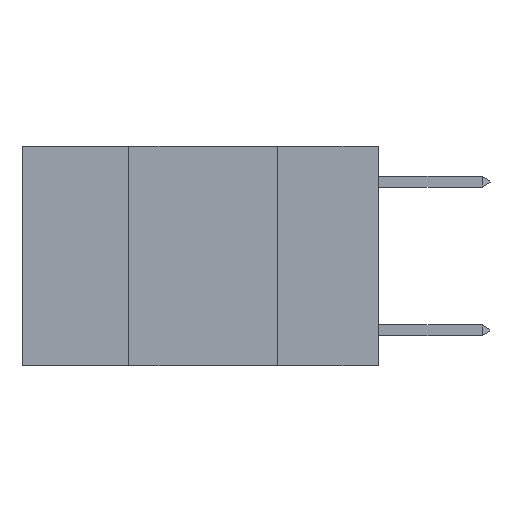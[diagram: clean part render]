
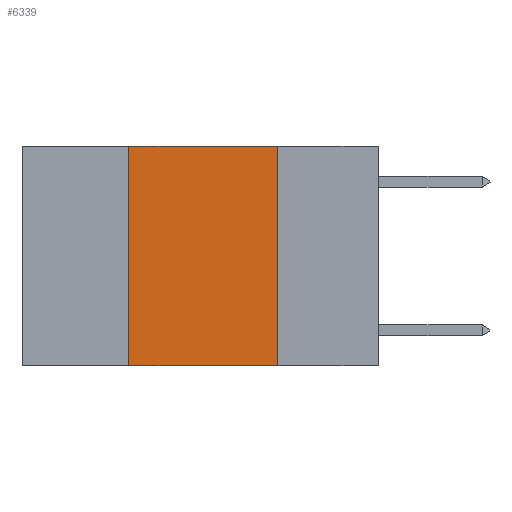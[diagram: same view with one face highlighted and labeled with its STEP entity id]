
A CAD part, left-side view. The second image highlights one B-rep face of the part: STEP entity #6339.
In plain terms, the highlighted planar face has unit normal (-1, 0, 0).
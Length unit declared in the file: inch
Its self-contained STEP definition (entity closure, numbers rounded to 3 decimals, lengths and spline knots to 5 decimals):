
#99 = CARTESIAN_POINT ( 'NONE',  ( 0., 0.6, -0.37 ) ) ;
#172 = EDGE_CURVE ( 'NONE', #1298, #14759, #4029, .T. ) ;
#753 = CARTESIAN_POINT ( 'NONE',  ( 0., 0.42, 0. ) ) ;
#875 = VECTOR ( 'NONE', #6077, 39.37008 ) ;
#1265 = ORIENTED_EDGE ( 'NONE', *, *, #14210, .F. ) ;
#1298 = VERTEX_POINT ( 'NONE', #15104 ) ;
#1406 = CARTESIAN_POINT ( 'NONE',  ( 0., 0.17, 0. ) ) ;
#1576 = VERTEX_POINT ( 'NONE', #1579 ) ;
#1579 = CARTESIAN_POINT ( 'NONE',  ( 0., 0.42, -0.37 ) ) ;
#1766 = LINE ( 'NONE', #99, #1829 ) ;
#1829 = VECTOR ( 'NONE', #12236, 39.37008 ) ;
#2841 = CARTESIAN_POINT ( 'NONE',  ( 0., 0.42, 0. ) ) ;
#3215 = DIRECTION ( 'NONE',  ( 1., 0., 0. ) ) ;
#4029 = LINE ( 'NONE', #1406, #13384 ) ;
#4341 = ORIENTED_EDGE ( 'NONE', *, *, #8536, .F. ) ;
#4842 = CARTESIAN_POINT ( 'NONE',  ( 0., 0.6, 0. ) ) ;
#5027 = EDGE_LOOP ( 'NONE', ( #6864, #1265, #4341, #5381 ) ) ;
#5381 = ORIENTED_EDGE ( 'NONE', *, *, #7319, .T. ) ;
#6077 = DIRECTION ( 'NONE',  ( 0., 0., 1. ) ) ;
#6339 = ADVANCED_FACE ( 'NONE', ( #7044 ), #12363, .F. ) ;
#6389 = CARTESIAN_POINT ( 'NONE',  ( 0., 0.17, -0.37 ) ) ;
#6864 = ORIENTED_EDGE ( 'NONE', *, *, #172, .F. ) ;
#7044 = FACE_OUTER_BOUND ( 'NONE', #5027, .T. ) ;
#7078 = AXIS2_PLACEMENT_3D ( 'NONE', #15132, #3215, #16095 ) ;
#7319 = EDGE_CURVE ( 'NONE', #1576, #14759, #1766, .T. ) ;
#8536 = EDGE_CURVE ( 'NONE', #1576, #14383, #12692, .T. ) ;
#10186 = DIRECTION ( 'NONE',  ( 0., -1., 0. ) ) ;
#11413 = LINE ( 'NONE', #4842, #16194 ) ;
#12236 = DIRECTION ( 'NONE',  ( 0., -1., 0. ) ) ;
#12363 = PLANE ( 'NONE',  #7078 ) ;
#12692 = LINE ( 'NONE', #753, #875 ) ;
#13345 = DIRECTION ( 'NONE',  ( 0., 0., -1. ) ) ;
#13384 = VECTOR ( 'NONE', #13345, 39.37008 ) ;
#14210 = EDGE_CURVE ( 'NONE', #14383, #1298, #11413, .T. ) ;
#14383 = VERTEX_POINT ( 'NONE', #2841 ) ;
#14759 = VERTEX_POINT ( 'NONE', #6389 ) ;
#15104 = CARTESIAN_POINT ( 'NONE',  ( 0., 0.17, 0. ) ) ;
#15132 = CARTESIAN_POINT ( 'NONE',  ( 0., 0.6, 0. ) ) ;
#16095 = DIRECTION ( 'NONE',  ( 0., 0., -1. ) ) ;
#16194 = VECTOR ( 'NONE', #10186, 39.37008 ) ;
